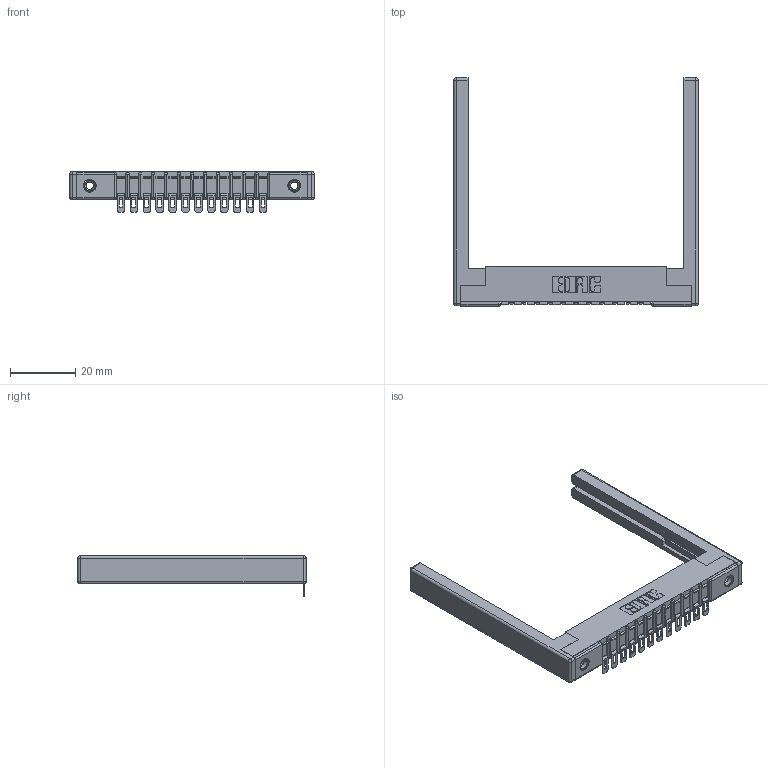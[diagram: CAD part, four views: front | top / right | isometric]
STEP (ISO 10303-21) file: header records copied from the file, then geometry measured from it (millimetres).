
FILE_DESCRIPTION (( 'STEP AP203' ), '1' );
FILE_NAME ('357-012-454-168.STEP', '2020-09-30T13:07:49', ( '' ), ( '' ), 'SwSTEP 2.0', 'SolidWorks 2020', '' );
FILE_SCHEMA (( 'CONFIG_CONTROL_DESIGN' ));
Length unit declared in the file: inch
Products named in the file (5): 307-290-002_554; 307 Part_.156 Dia Mounting Holes; 357-012-454-168; 345-250-001_345-250-001-102; 307-220-068
Assembly tree (17 placements, depth 2):
  357-012-454-168
    307 Part_.156 Dia Mounting Holes
    307-290-002_554  x12
    307-220-068  x2
    345-250-001_345-250-001-102  x2
Bounding box: 74.98 x 69.98 x 12.52 mm (x, y, z)
Volume: 9508 mm3; surface area: 12515.6 mm2
Topology: 17 solids, 17 shells, 1257 faces, 3749 edges, 2442 vertices
Faces by surface type: plane 710, cylinder 497, sphere 34, cone 12, torus 4
Entity records: 17710 total; most frequent: CARTESIAN_POINT 2947, ORIENTED_EDGE 2926, DIRECTION 2901, EDGE_CURVE 1463, LINE 1097, VECTOR 1097, VERTEX_POINT 948, AXIS2_PLACEMENT_3D 902
